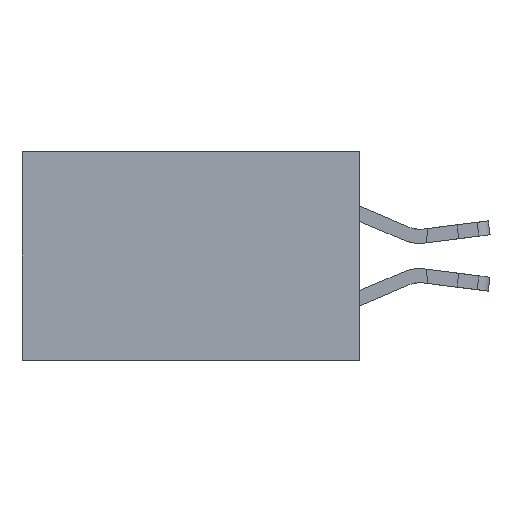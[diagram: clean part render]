
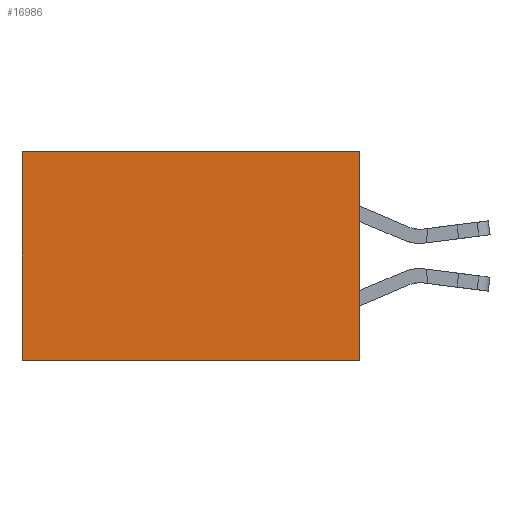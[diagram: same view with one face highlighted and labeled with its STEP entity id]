
A CAD part, left-side view. The second image highlights one B-rep face of the part: STEP entity #16986.
In plain terms, the highlighted planar face has unit normal (-1, 0, 0).
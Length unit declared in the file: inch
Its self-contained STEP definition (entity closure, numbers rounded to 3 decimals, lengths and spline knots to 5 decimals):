
#45 = VECTOR ( 'NONE', #11824, 39.37008 ) ;
#492 = LINE ( 'NONE', #1743, #25394 ) ;
#1394 = VECTOR ( 'NONE', #26492, 39.37008 ) ;
#1570 = LINE ( 'NONE', #9495, #45 ) ;
#1743 = CARTESIAN_POINT ( 'NONE',  ( 0.2875, 0., 0. ) ) ;
#2753 = CARTESIAN_POINT ( 'NONE',  ( 0.2875, 0.6, 0. ) ) ;
#4429 = AXIS2_PLACEMENT_3D ( 'NONE', #11617, #28294, #13999 ) ;
#4740 = EDGE_CURVE ( 'NONE', #9250, #17020, #7894, .T. ) ;
#6890 = CARTESIAN_POINT ( 'NONE',  ( 0.2875, 0., -0.37 ) ) ;
#7830 = CARTESIAN_POINT ( 'NONE',  ( 0.2875, 0., 0. ) ) ;
#7894 = LINE ( 'NONE', #21752, #1394 ) ;
#9094 = DIRECTION ( 'NONE',  ( 0., 1., 0. ) ) ;
#9250 = VERTEX_POINT ( 'NONE', #7830 ) ;
#9495 = CARTESIAN_POINT ( 'NONE',  ( 0.2875, 0.6, 0. ) ) ;
#9887 = FACE_OUTER_BOUND ( 'NONE', #26618, .T. ) ;
#11415 = PLANE ( 'NONE',  #4429 ) ;
#11617 = CARTESIAN_POINT ( 'NONE',  ( 0.2875, 0., 0. ) ) ;
#11824 = DIRECTION ( 'NONE',  ( 0., 0., -1. ) ) ;
#13522 = VERTEX_POINT ( 'NONE', #19245 ) ;
#13999 = DIRECTION ( 'NONE',  ( 0., 0., -1. ) ) ;
#14233 = VERTEX_POINT ( 'NONE', #2753 ) ;
#16986 = ADVANCED_FACE ( 'NONE', ( #9887 ), #11415, .F. ) ;
#17020 = VERTEX_POINT ( 'NONE', #6890 ) ;
#19245 = CARTESIAN_POINT ( 'NONE',  ( 0.2875, 0.6, -0.37 ) ) ;
#20754 = ORIENTED_EDGE ( 'NONE', *, *, #26439, .F. ) ;
#21537 = CARTESIAN_POINT ( 'NONE',  ( 0.2875, 0., -0.37 ) ) ;
#21752 = CARTESIAN_POINT ( 'NONE',  ( 0.2875, 0., 0. ) ) ;
#21938 = EDGE_CURVE ( 'NONE', #9250, #14233, #492, .T. ) ;
#23312 = EDGE_CURVE ( 'NONE', #14233, #13522, #1570, .T. ) ;
#25394 = VECTOR ( 'NONE', #9094, 39.37008 ) ;
#26439 = EDGE_CURVE ( 'NONE', #17020, #13522, #29905, .T. ) ;
#26492 = DIRECTION ( 'NONE',  ( 0., 0., -1. ) ) ;
#26618 = EDGE_LOOP ( 'NONE', ( #30003, #20754, #30775, #28145 ) ) ;
#28145 = ORIENTED_EDGE ( 'NONE', *, *, #21938, .T. ) ;
#28294 = DIRECTION ( 'NONE',  ( 1., 0., 0. ) ) ;
#29143 = VECTOR ( 'NONE', #31023, 39.37008 ) ;
#29905 = LINE ( 'NONE', #21537, #29143 ) ;
#30003 = ORIENTED_EDGE ( 'NONE', *, *, #23312, .T. ) ;
#30775 = ORIENTED_EDGE ( 'NONE', *, *, #4740, .F. ) ;
#31023 = DIRECTION ( 'NONE',  ( 0., 1., 0. ) ) ;
